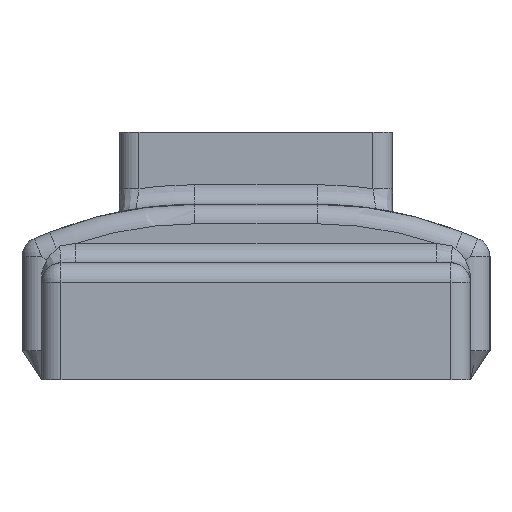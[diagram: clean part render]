
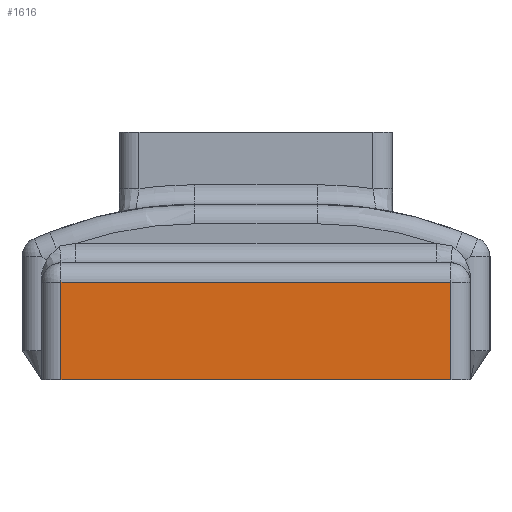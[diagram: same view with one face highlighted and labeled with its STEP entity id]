
A CAD part, left-side view. The second image highlights one B-rep face of the part: STEP entity #1616.
In plain terms, the highlighted planar face has unit normal (-1, 0, 0).
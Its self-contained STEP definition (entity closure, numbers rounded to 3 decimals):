
#113=PLANE('',#1745);
#150=FACE_OUTER_BOUND('',#256,.T.);
#256=EDGE_LOOP('',(#1091,#1092,#1093,#1094));
#370=LINE('',#2447,#474);
#372=LINE('',#2455,#476);
#373=LINE('',#2460,#477);
#375=LINE('',#2469,#479);
#474=VECTOR('',#1942,10.);
#476=VECTOR('',#1950,10.);
#477=VECTOR('',#1955,10.);
#479=VECTOR('',#1969,10.);
#677=VERTEX_POINT('',#2440);
#680=VERTEX_POINT('',#2445);
#683=VERTEX_POINT('',#2453);
#685=VERTEX_POINT('',#2458);
#826=EDGE_CURVE('',#680,#677,#370,.T.);
#830=EDGE_CURVE('',#683,#680,#372,.T.);
#832=EDGE_CURVE('',#685,#683,#373,.T.);
#837=EDGE_CURVE('',#677,#685,#375,.T.);
#1091=ORIENTED_EDGE('',*,*,#826,.F.);
#1092=ORIENTED_EDGE('',*,*,#830,.F.);
#1093=ORIENTED_EDGE('',*,*,#832,.F.);
#1094=ORIENTED_EDGE('',*,*,#837,.F.);
#1616=ADVANCED_FACE('',(#150),#113,.T.);
#1745=AXIS2_PLACEMENT_3D('',#2468,#1967,#1968);
#1942=DIRECTION('',(0.,0.,-1.));
#1950=DIRECTION('',(0.,-1.,0.));
#1955=DIRECTION('',(0.,0.,1.));
#1967=DIRECTION('center_axis',(-1.,0.,0.));
#1968=DIRECTION('ref_axis',(0.,-1.,0.));
#1969=DIRECTION('',(0.,1.,0.));
#2440=CARTESIAN_POINT('',(27.5,-55.,0.));
#2445=CARTESIAN_POINT('',(27.5,-55.,2.5));
#2447=CARTESIAN_POINT('',(27.5,-55.,0.));
#2453=CARTESIAN_POINT('',(27.5,-45.,2.5));
#2455=CARTESIAN_POINT('',(27.5,-47.25,2.5));
#2458=CARTESIAN_POINT('',(27.5,-45.,0.));
#2460=CARTESIAN_POINT('',(27.5,-45.,0.));
#2468=CARTESIAN_POINT('Origin',(27.5,-44.5,0.));
#2469=CARTESIAN_POINT('',(27.5,-47.25,0.));
